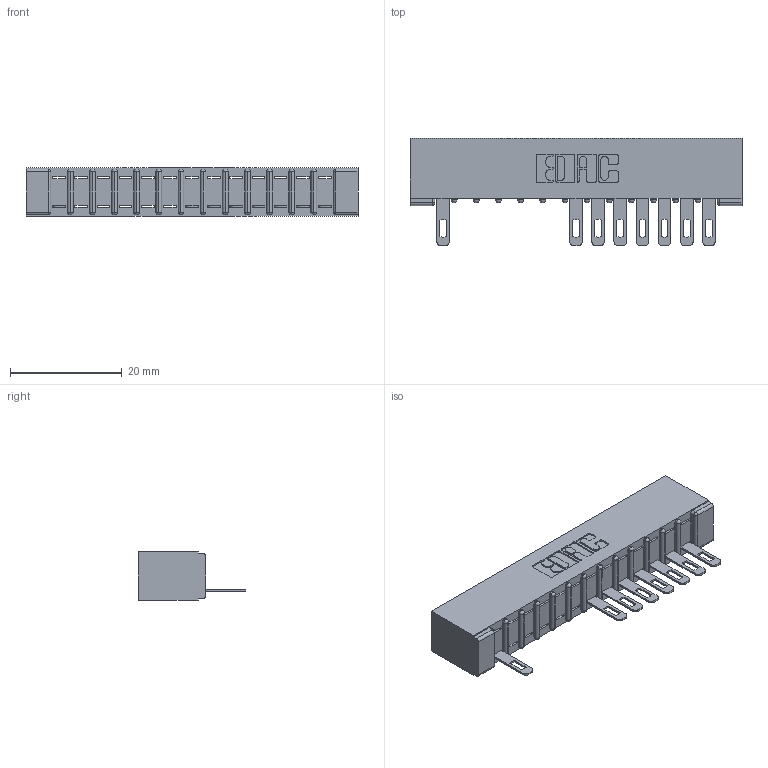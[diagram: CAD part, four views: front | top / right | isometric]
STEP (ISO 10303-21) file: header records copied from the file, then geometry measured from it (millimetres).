
FILE_DESCRIPTION (( 'STEP AP203' ), '1' );
FILE_NAME ('307-013-505-101.STEP', '2018-08-02T23:28:49', ( '' ), ( '' ), 'SwSTEP 2.0', 'SolidWorks 2016', '' );
FILE_SCHEMA (( 'CONFIG_CONTROL_DESIGN' ));
Length unit declared in the file: inch
Products named in the file (3): 307 Part_No Mounting Lugs; 307-290-001_505; 307-013-505-101
Assembly tree (9 placements, depth 2):
  307-013-505-101
    307 Part_No Mounting Lugs
    307-290-001_505  x8
Bounding box: 59.39 x 19.18 x 8.71 mm (x, y, z)
Volume: 3908.8 mm3; surface area: 5658.5 mm2
Topology: 9 solids, 9 shells, 672 faces, 1915 edges, 1226 vertices
Faces by surface type: plane 414, cylinder 230, sphere 28
Entity records: 14256 total; most frequent: CARTESIAN_POINT 2411, ORIENTED_EDGE 2402, DIRECTION 2357, EDGE_CURVE 1201, LINE 909, VECTOR 909, VERTEX_POINT 778, AXIS2_PLACEMENT_3D 724
